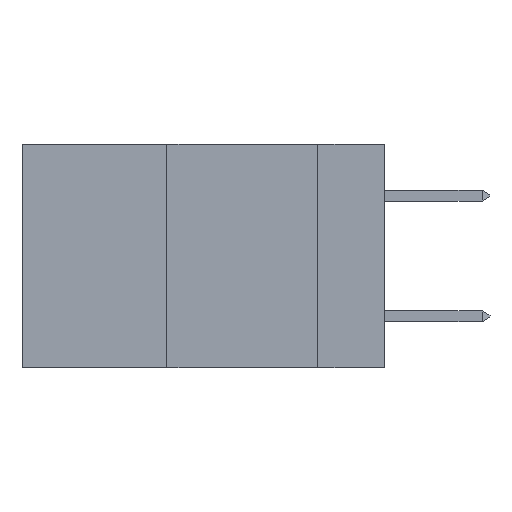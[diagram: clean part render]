
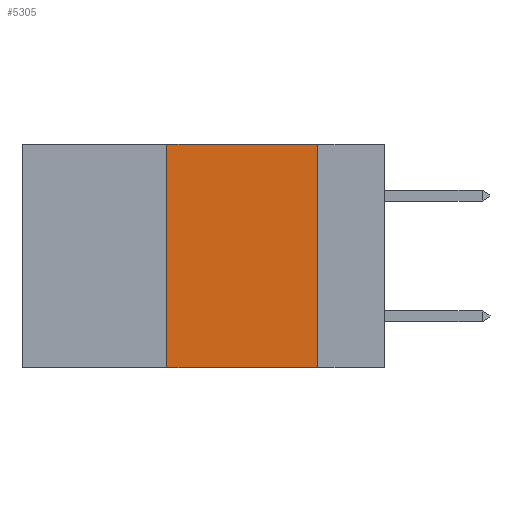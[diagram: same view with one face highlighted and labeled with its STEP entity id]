
A CAD part, left-side view. The second image highlights one B-rep face of the part: STEP entity #5305.
In plain terms, the highlighted planar face has unit normal (-1, 0, 0).
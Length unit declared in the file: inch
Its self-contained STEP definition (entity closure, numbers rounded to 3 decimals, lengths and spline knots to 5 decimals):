
#160 = DIRECTION ( 'NONE',  ( 0., -1., 0. ) ) ;
#271 = LINE ( 'NONE', #10899, #733 ) ;
#381 = VECTOR ( 'NONE', #1598, 39.37008 ) ;
#520 = CARTESIAN_POINT ( 'NONE',  ( 0., 0.36, -0.37 ) ) ;
#628 = VECTOR ( 'NONE', #160, 39.37008 ) ;
#733 = VECTOR ( 'NONE', #10949, 39.37008 ) ;
#777 = CARTESIAN_POINT ( 'NONE',  ( 0., 0.6, 0. ) ) ;
#862 = EDGE_CURVE ( 'NONE', #6745, #2312, #8154, .T. ) ;
#920 = CARTESIAN_POINT ( 'NONE',  ( 0., 0.6, -0.37 ) ) ;
#1598 = DIRECTION ( 'NONE',  ( 0., 0., -1. ) ) ;
#2312 = VERTEX_POINT ( 'NONE', #7358 ) ;
#2717 = EDGE_CURVE ( 'NONE', #4069, #10690, #271, .T. ) ;
#3255 = ORIENTED_EDGE ( 'NONE', *, *, #862, .T. ) ;
#3327 = EDGE_CURVE ( 'NONE', #10690, #2312, #11278, .T. ) ;
#3373 = VECTOR ( 'NONE', #6029, 39.37008 ) ;
#3465 = EDGE_CURVE ( 'NONE', #6745, #4069, #6823, .T. ) ;
#3684 = CARTESIAN_POINT ( 'NONE',  ( 0., 0.36, 0. ) ) ;
#4069 = VERTEX_POINT ( 'NONE', #3684 ) ;
#4274 = PLANE ( 'NONE',  #8582 ) ;
#4398 = DIRECTION ( 'NONE',  ( 1., 0., 0. ) ) ;
#5305 = ADVANCED_FACE ( 'NONE', ( #10472 ), #4274, .F. ) ;
#5904 = CARTESIAN_POINT ( 'NONE',  ( 0., 0.11, 0. ) ) ;
#6029 = DIRECTION ( 'NONE',  ( 0., 0., 1. ) ) ;
#6669 = ORIENTED_EDGE ( 'NONE', *, *, #2717, .F. ) ;
#6745 = VERTEX_POINT ( 'NONE', #520 ) ;
#6823 = LINE ( 'NONE', #10470, #3373 ) ;
#7152 = ORIENTED_EDGE ( 'NONE', *, *, #3327, .F. ) ;
#7358 = CARTESIAN_POINT ( 'NONE',  ( 0., 0.11, -0.37 ) ) ;
#7823 = DIRECTION ( 'NONE',  ( 0., 0., -1. ) ) ;
#8154 = LINE ( 'NONE', #920, #628 ) ;
#8582 = AXIS2_PLACEMENT_3D ( 'NONE', #777, #4398, #7823 ) ;
#8660 = EDGE_LOOP ( 'NONE', ( #7152, #6669, #11355, #3255 ) ) ;
#10470 = CARTESIAN_POINT ( 'NONE',  ( 0., 0.36, 0. ) ) ;
#10472 = FACE_OUTER_BOUND ( 'NONE', #8660, .T. ) ;
#10690 = VERTEX_POINT ( 'NONE', #11521 ) ;
#10899 = CARTESIAN_POINT ( 'NONE',  ( 0., 0.6, 0. ) ) ;
#10949 = DIRECTION ( 'NONE',  ( 0., -1., 0. ) ) ;
#11278 = LINE ( 'NONE', #5904, #381 ) ;
#11355 = ORIENTED_EDGE ( 'NONE', *, *, #3465, .F. ) ;
#11521 = CARTESIAN_POINT ( 'NONE',  ( 0., 0.11, 0. ) ) ;
